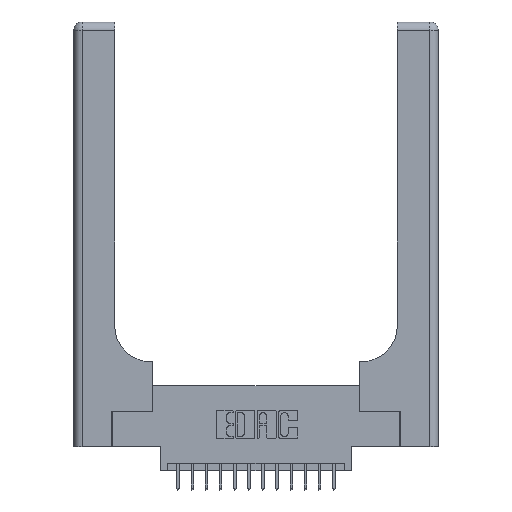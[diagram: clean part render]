
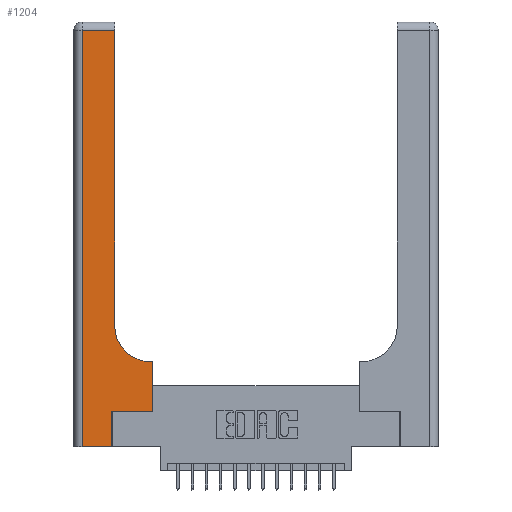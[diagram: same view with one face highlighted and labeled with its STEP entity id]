
A CAD part, top view. The second image highlights one B-rep face of the part: STEP entity #1204.
In plain terms, the highlighted planar face has unit normal (0, 0, 1).
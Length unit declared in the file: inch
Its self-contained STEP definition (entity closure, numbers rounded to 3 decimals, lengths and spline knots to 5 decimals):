
#34 = CARTESIAN_POINT ( 'NONE',  ( 0.269, 0.25, 0.37 ) ) ;
#116 = LINE ( 'NONE', #10393, #5413 ) ;
#385 = DIRECTION ( 'NONE',  ( 0., 0., -1. ) ) ;
#720 = ORIENTED_EDGE ( 'NONE', *, *, #18475, .T. ) ;
#808 = VERTEX_POINT ( 'NONE', #5920 ) ;
#1204 = ADVANCED_FACE ( 'NONE', ( #8024 ), #3423, .F. ) ;
#1518 = DIRECTION ( 'NONE',  ( -1., 0., 0. ) ) ;
#1579 = CARTESIAN_POINT ( 'NONE',  ( 0.269, 0., 0.37 ) ) ;
#1996 = ORIENTED_EDGE ( 'NONE', *, *, #18088, .T. ) ;
#2371 = LINE ( 'NONE', #8254, #15165 ) ;
#2491 = CARTESIAN_POINT ( 'NONE',  ( 0.5415, 0.6, 0.37 ) ) ;
#2947 = CARTESIAN_POINT ( 'NONE',  ( 0.06, 2.94, 0.37 ) ) ;
#3192 = AXIS2_PLACEMENT_3D ( 'NONE', #7778, #385, #14805 ) ;
#3400 = EDGE_CURVE ( 'NONE', #808, #10659, #18825, .T. ) ;
#3423 = PLANE ( 'NONE',  #12963 ) ;
#3904 = EDGE_CURVE ( 'NONE', #6953, #4925, #116, .T. ) ;
#3962 = VECTOR ( 'NONE', #11259, 39.37008 ) ;
#4106 = DIRECTION ( 'NONE',  ( 0., 1., 0. ) ) ;
#4261 = LINE ( 'NONE', #14245, #11005 ) ;
#4350 = DIRECTION ( 'NONE',  ( 1., 0., 0. ) ) ;
#4381 = ORIENTED_EDGE ( 'NONE', *, *, #3904, .T. ) ;
#4925 = VERTEX_POINT ( 'NONE', #6807 ) ;
#4965 = DIRECTION ( 'NONE',  ( 0., 0., -1. ) ) ;
#5338 = CARTESIAN_POINT ( 'NONE',  ( 0.2915, 0.85, 0.37 ) ) ;
#5413 = VECTOR ( 'NONE', #16123, 39.37008 ) ;
#5807 = CARTESIAN_POINT ( 'NONE',  ( 0., 0., 0.37 ) ) ;
#5908 = DIRECTION ( 'NONE',  ( 1., 0., 0. ) ) ;
#5920 = CARTESIAN_POINT ( 'NONE',  ( 0.06, 0., 0.37 ) ) ;
#6186 = CARTESIAN_POINT ( 'NONE',  ( 0.06, 3., 0.37 ) ) ;
#6393 = ORIENTED_EDGE ( 'NONE', *, *, #15590, .T. ) ;
#6807 = CARTESIAN_POINT ( 'NONE',  ( 0.5585, 0.6, 0.37 ) ) ;
#6953 = VERTEX_POINT ( 'NONE', #18029 ) ;
#7088 = EDGE_CURVE ( 'NONE', #4925, #15299, #17809, .T. ) ;
#7433 = VERTEX_POINT ( 'NONE', #2947 ) ;
#7778 = CARTESIAN_POINT ( 'NONE',  ( 0.5415, 0.85, 0.37 ) ) ;
#8024 = FACE_OUTER_BOUND ( 'NONE', #14840, .T. ) ;
#8254 = CARTESIAN_POINT ( 'NONE',  ( 0.269, 0., 0.37 ) ) ;
#8917 = VECTOR ( 'NONE', #5908, 39.37008 ) ;
#9143 = DIRECTION ( 'NONE',  ( 0., -1., 0. ) ) ;
#9246 = EDGE_CURVE ( 'NONE', #15299, #12865, #18081, .T. ) ;
#10282 = VECTOR ( 'NONE', #4350, 39.37008 ) ;
#10393 = CARTESIAN_POINT ( 'NONE',  ( 0.5585, 0.25, 0.37 ) ) ;
#10659 = VERTEX_POINT ( 'NONE', #1579 ) ;
#10693 = CARTESIAN_POINT ( 'NONE',  ( 0.269, 0.25, 0.37 ) ) ;
#11005 = VECTOR ( 'NONE', #11341, 39.37008 ) ;
#11249 = ORIENTED_EDGE ( 'NONE', *, *, #18451, .T. ) ;
#11259 = DIRECTION ( 'NONE',  ( -1., 0., 0. ) ) ;
#11341 = DIRECTION ( 'NONE',  ( 0., 1., 0. ) ) ;
#11438 = LINE ( 'NONE', #34, #8917 ) ;
#11579 = VERTEX_POINT ( 'NONE', #10693 ) ;
#12447 = ORIENTED_EDGE ( 'NONE', *, *, #9246, .T. ) ;
#12865 = VERTEX_POINT ( 'NONE', #5338 ) ;
#12873 = ORIENTED_EDGE ( 'NONE', *, *, #15170, .T. ) ;
#12963 = AXIS2_PLACEMENT_3D ( 'NONE', #15104, #4965, #15014 ) ;
#13412 = CARTESIAN_POINT ( 'NONE',  ( 0.2915, 0.6, 0.37 ) ) ;
#13534 = LINE ( 'NONE', #6186, #17364 ) ;
#14071 = LINE ( 'NONE', #17115, #3962 ) ;
#14245 = CARTESIAN_POINT ( 'NONE',  ( 0.2915, 3., 0.37 ) ) ;
#14805 = DIRECTION ( 'NONE',  ( 1., 0., 0. ) ) ;
#14840 = EDGE_LOOP ( 'NONE', ( #1996, #12873, #720, #17028, #6393, #11249, #4381, #18223, #12447 ) ) ;
#14852 = VECTOR ( 'NONE', #1518, 39.37008 ) ;
#15014 = DIRECTION ( 'NONE',  ( -1., 0., 0. ) ) ;
#15104 = CARTESIAN_POINT ( 'NONE',  ( 0., 3., 0.37 ) ) ;
#15165 = VECTOR ( 'NONE', #4106, 39.37008 ) ;
#15170 = EDGE_CURVE ( 'NONE', #18477, #7433, #14071, .T. ) ;
#15299 = VERTEX_POINT ( 'NONE', #2491 ) ;
#15590 = EDGE_CURVE ( 'NONE', #10659, #11579, #2371, .T. ) ;
#16117 = CARTESIAN_POINT ( 'NONE',  ( 0.2915, 2.94, 0.37 ) ) ;
#16123 = DIRECTION ( 'NONE',  ( 0., 1., 0. ) ) ;
#17028 = ORIENTED_EDGE ( 'NONE', *, *, #3400, .T. ) ;
#17115 = CARTESIAN_POINT ( 'NONE',  ( 0., 2.94, 0.37 ) ) ;
#17364 = VECTOR ( 'NONE', #9143, 39.37008 ) ;
#17809 = LINE ( 'NONE', #13412, #14852 ) ;
#18029 = CARTESIAN_POINT ( 'NONE',  ( 0.5585, 0.25, 0.37 ) ) ;
#18081 = CIRCLE ( 'NONE', #3192, 0.25 ) ;
#18088 = EDGE_CURVE ( 'NONE', #12865, #18477, #4261, .T. ) ;
#18223 = ORIENTED_EDGE ( 'NONE', *, *, #7088, .T. ) ;
#18451 = EDGE_CURVE ( 'NONE', #11579, #6953, #11438, .T. ) ;
#18475 = EDGE_CURVE ( 'NONE', #7433, #808, #13534, .T. ) ;
#18477 = VERTEX_POINT ( 'NONE', #16117 ) ;
#18825 = LINE ( 'NONE', #5807, #10282 ) ;
